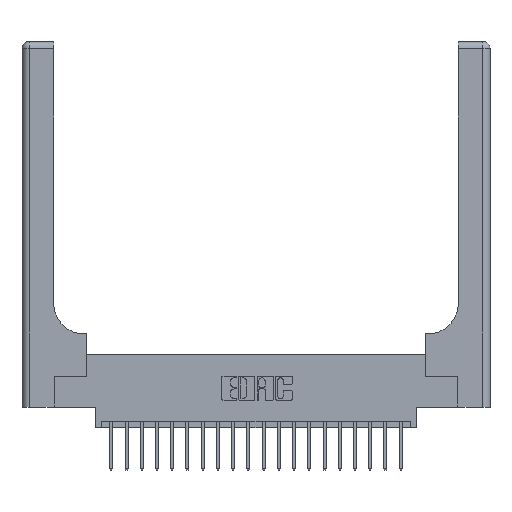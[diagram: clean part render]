
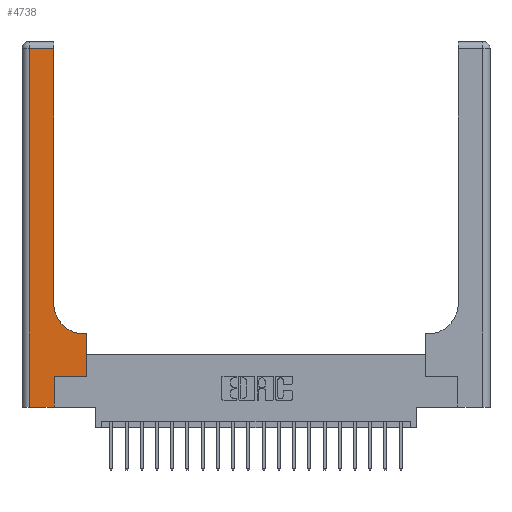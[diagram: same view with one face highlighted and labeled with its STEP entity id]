
A CAD part, top view. The second image highlights one B-rep face of the part: STEP entity #4738.
In plain terms, the highlighted planar face has unit normal (0, 0, 1).
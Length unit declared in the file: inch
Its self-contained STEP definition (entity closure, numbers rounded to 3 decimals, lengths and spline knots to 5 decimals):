
#231 = LINE ( 'NONE', #16989, #20248 ) ;
#289 = CARTESIAN_POINT ( 'NONE',  ( 0.06, 3., 0.37 ) ) ;
#293 = EDGE_CURVE ( 'NONE', #19234, #20658, #231, .T. ) ;
#556 = ORIENTED_EDGE ( 'NONE', *, *, #11952, .T. ) ;
#664 = VECTOR ( 'NONE', #7008, 39.37008 ) ;
#804 = CARTESIAN_POINT ( 'NONE',  ( 0.51, 0.6, 0.37 ) ) ;
#1005 = ORIENTED_EDGE ( 'NONE', *, *, #17398, .T. ) ;
#1156 = VECTOR ( 'NONE', #14678, 39.37008 ) ;
#1210 = EDGE_CURVE ( 'NONE', #2350, #15673, #8642, .T. ) ;
#1211 = ORIENTED_EDGE ( 'NONE', *, *, #16483, .T. ) ;
#2350 = VERTEX_POINT ( 'NONE', #6906 ) ;
#2615 = VERTEX_POINT ( 'NONE', #13053 ) ;
#2651 = DIRECTION ( 'NONE',  ( -1., 0., 0. ) ) ;
#2892 = VECTOR ( 'NONE', #9773, 39.37008 ) ;
#3065 = ORIENTED_EDGE ( 'NONE', *, *, #21011, .T. ) ;
#3089 = EDGE_CURVE ( 'NONE', #15673, #16425, #20087, .T. ) ;
#3243 = CARTESIAN_POINT ( 'NONE',  ( 0.528, 0.25, 0.37 ) ) ;
#4336 = VECTOR ( 'NONE', #18702, 39.37008 ) ;
#4738 = ADVANCED_FACE ( 'NONE', ( #13534 ), #15057, .F. ) ;
#4973 = CARTESIAN_POINT ( 'NONE',  ( 0., 0., 0.37 ) ) ;
#4992 = ORIENTED_EDGE ( 'NONE', *, *, #11617, .T. ) ;
#5635 = CIRCLE ( 'NONE', #20058, 0.25 ) ;
#6906 = CARTESIAN_POINT ( 'NONE',  ( 0.06, 2.94, 0.37 ) ) ;
#7008 = DIRECTION ( 'NONE',  ( 0., -1., 0. ) ) ;
#7250 = EDGE_LOOP ( 'NONE', ( #4992, #3065, #14847, #15631, #1005, #10514, #11406, #1211, #556 ) ) ;
#7266 = LINE ( 'NONE', #17194, #9228 ) ;
#7729 = CARTESIAN_POINT ( 'NONE',  ( 0.06, 0., 0.37 ) ) ;
#7856 = CARTESIAN_POINT ( 'NONE',  ( 0.265, 0.25, 0.37 ) ) ;
#7965 = DIRECTION ( 'NONE',  ( 0., 0., -1. ) ) ;
#8547 = CARTESIAN_POINT ( 'NONE',  ( 0., 3., 0.37 ) ) ;
#8642 = LINE ( 'NONE', #289, #664 ) ;
#8783 = DIRECTION ( 'NONE',  ( 0., 1., 0. ) ) ;
#9032 = VERTEX_POINT ( 'NONE', #16693 ) ;
#9228 = VECTOR ( 'NONE', #8783, 39.37008 ) ;
#9773 = DIRECTION ( 'NONE',  ( 1., 0., 0. ) ) ;
#10196 = DIRECTION ( 'NONE',  ( 0., 0., -1. ) ) ;
#10514 = ORIENTED_EDGE ( 'NONE', *, *, #17049, .T. ) ;
#11127 = CARTESIAN_POINT ( 'NONE',  ( 0., 2.94, 0.37 ) ) ;
#11265 = DIRECTION ( 'NONE',  ( 0., 1., 0. ) ) ;
#11334 = CARTESIAN_POINT ( 'NONE',  ( 0.265, 0.25, 0.37 ) ) ;
#11406 = ORIENTED_EDGE ( 'NONE', *, *, #293, .T. ) ;
#11617 = EDGE_CURVE ( 'NONE', #9032, #2615, #18162, .T. ) ;
#11952 = EDGE_CURVE ( 'NONE', #13292, #9032, #5635, .T. ) ;
#12696 = LINE ( 'NONE', #11127, #20645 ) ;
#12795 = VERTEX_POINT ( 'NONE', #7856 ) ;
#13053 = CARTESIAN_POINT ( 'NONE',  ( 0.26, 2.94, 0.37 ) ) ;
#13164 = CARTESIAN_POINT ( 'NONE',  ( 0.51, 0.85, 0.37 ) ) ;
#13191 = CARTESIAN_POINT ( 'NONE',  ( 0.265, 0., 0.37 ) ) ;
#13292 = VERTEX_POINT ( 'NONE', #804 ) ;
#13534 = FACE_OUTER_BOUND ( 'NONE', #7250, .T. ) ;
#14678 = DIRECTION ( 'NONE',  ( 1., 0., 0. ) ) ;
#14707 = DIRECTION ( 'NONE',  ( 1., 0., 0. ) ) ;
#14847 = ORIENTED_EDGE ( 'NONE', *, *, #1210, .T. ) ;
#15057 = PLANE ( 'NONE',  #21051 ) ;
#15631 = ORIENTED_EDGE ( 'NONE', *, *, #3089, .T. ) ;
#15673 = VERTEX_POINT ( 'NONE', #7729 ) ;
#16203 = LINE ( 'NONE', #11334, #2892 ) ;
#16425 = VERTEX_POINT ( 'NONE', #13191 ) ;
#16483 = EDGE_CURVE ( 'NONE', #20658, #13292, #17380, .T. ) ;
#16693 = CARTESIAN_POINT ( 'NONE',  ( 0.26, 0.85, 0.37 ) ) ;
#16989 = CARTESIAN_POINT ( 'NONE',  ( 0.528, 0.25, 0.37 ) ) ;
#17049 = EDGE_CURVE ( 'NONE', #12795, #19234, #16203, .T. ) ;
#17194 = CARTESIAN_POINT ( 'NONE',  ( 0.265, 0., 0.37 ) ) ;
#17380 = LINE ( 'NONE', #17489, #4336 ) ;
#17398 = EDGE_CURVE ( 'NONE', #16425, #12795, #7266, .T. ) ;
#17489 = CARTESIAN_POINT ( 'NONE',  ( 0.26, 0.6, 0.37 ) ) ;
#18162 = LINE ( 'NONE', #19618, #18642 ) ;
#18642 = VECTOR ( 'NONE', #21710, 39.37008 ) ;
#18702 = DIRECTION ( 'NONE',  ( -1., 0., 0. ) ) ;
#18712 = DIRECTION ( 'NONE',  ( -1., 0., 0. ) ) ;
#19234 = VERTEX_POINT ( 'NONE', #3243 ) ;
#19618 = CARTESIAN_POINT ( 'NONE',  ( 0.26, 3., 0.37 ) ) ;
#20058 = AXIS2_PLACEMENT_3D ( 'NONE', #13164, #7965, #14707 ) ;
#20087 = LINE ( 'NONE', #4973, #1156 ) ;
#20248 = VECTOR ( 'NONE', #11265, 39.37008 ) ;
#20645 = VECTOR ( 'NONE', #2651, 39.37008 ) ;
#20658 = VERTEX_POINT ( 'NONE', #21255 ) ;
#21011 = EDGE_CURVE ( 'NONE', #2615, #2350, #12696, .T. ) ;
#21051 = AXIS2_PLACEMENT_3D ( 'NONE', #8547, #10196, #18712 ) ;
#21255 = CARTESIAN_POINT ( 'NONE',  ( 0.528, 0.6, 0.37 ) ) ;
#21710 = DIRECTION ( 'NONE',  ( 0., 1., 0. ) ) ;
